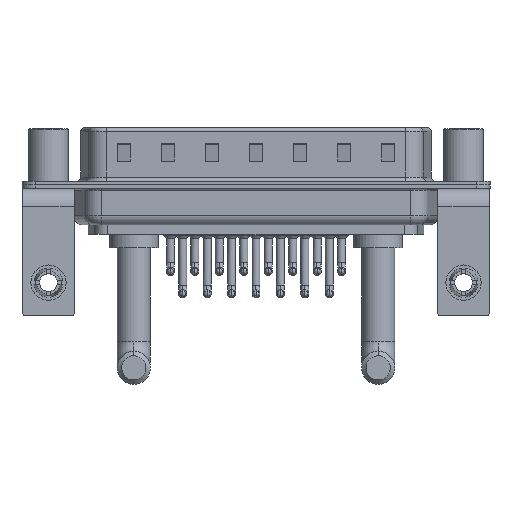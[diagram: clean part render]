
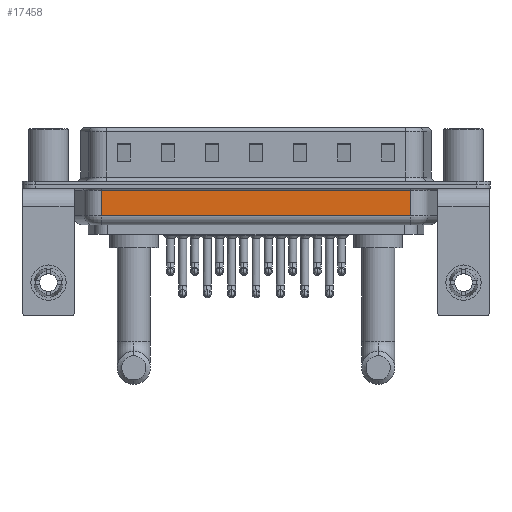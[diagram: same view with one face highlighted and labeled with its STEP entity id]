
A CAD part, front view. The second image highlights one B-rep face of the part: STEP entity #17458.
In plain terms, the highlighted planar face has unit normal (0, -1, 0).
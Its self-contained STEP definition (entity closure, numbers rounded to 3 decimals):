
#133 = LINE ( 'NONE', #23718, #7678 ) ;
#480 = CARTESIAN_POINT ( 'NONE',  ( 6.006, -5.35, -4.5 ) ) ;
#518 = CARTESIAN_POINT ( 'NONE',  ( 41.044, -5.35, -3.5 ) ) ;
#692 = VERTEX_POINT ( 'NONE', #19243 ) ;
#1671 = VECTOR ( 'NONE', #14717, 1000. ) ;
#2708 = VERTEX_POINT ( 'NONE', #16312 ) ;
#3236 = AXIS2_PLACEMENT_3D ( 'NONE', #26106, #8802, #17519 ) ;
#3366 = EDGE_LOOP ( 'NONE', ( #18526, #5207, #11233, #5234 ) ) ;
#4240 = FACE_OUTER_BOUND ( 'NONE', #3366, .T. ) ;
#4291 = DIRECTION ( 'NONE',  ( 1., 0., 0. ) ) ;
#5139 = VERTEX_POINT ( 'NONE', #518 ) ;
#5207 = ORIENTED_EDGE ( 'NONE', *, *, #7796, .T. ) ;
#5234 = ORIENTED_EDGE ( 'NONE', *, *, #7615, .T. ) ;
#6622 = VERTEX_POINT ( 'NONE', #27382 ) ;
#7615 = EDGE_CURVE ( 'NONE', #2708, #692, #10151, .T. ) ;
#7678 = VECTOR ( 'NONE', #4291, 1000. ) ;
#7796 = EDGE_CURVE ( 'NONE', #6622, #5139, #133, .T. ) ;
#7885 = CARTESIAN_POINT ( 'NONE',  ( 41.044, -5.35, -4.5 ) ) ;
#8601 = DIRECTION ( 'NONE',  ( 0., 0., 1. ) ) ;
#8802 = DIRECTION ( 'NONE',  ( 0., 1., 0. ) ) ;
#10151 = LINE ( 'NONE', #21297, #1671 ) ;
#10825 = PLANE ( 'NONE',  #3236 ) ;
#11233 = ORIENTED_EDGE ( 'NONE', *, *, #19568, .T. ) ;
#14048 = LINE ( 'NONE', #480, #23094 ) ;
#14717 = DIRECTION ( 'NONE',  ( -1., 0., 0. ) ) ;
#16312 = CARTESIAN_POINT ( 'NONE',  ( 41.044, -5.35, -0.65 ) ) ;
#17458 = ADVANCED_FACE ( 'NONE', ( #4240 ), #10825, .F. ) ;
#17519 = DIRECTION ( 'NONE',  ( 0., 0., 1. ) ) ;
#18526 = ORIENTED_EDGE ( 'NONE', *, *, #23560, .F. ) ;
#19243 = CARTESIAN_POINT ( 'NONE',  ( 6.006, -5.35, -0.65 ) ) ;
#19258 = VECTOR ( 'NONE', #8601, 1000. ) ;
#19568 = EDGE_CURVE ( 'NONE', #5139, #2708, #23016, .T. ) ;
#21297 = CARTESIAN_POINT ( 'NONE',  ( 6.006, -5.35, -0.65 ) ) ;
#22760 = DIRECTION ( 'NONE',  ( 0., 0., 1. ) ) ;
#23016 = LINE ( 'NONE', #7885, #19258 ) ;
#23094 = VECTOR ( 'NONE', #22760, 1000. ) ;
#23560 = EDGE_CURVE ( 'NONE', #6622, #692, #14048, .T. ) ;
#23718 = CARTESIAN_POINT ( 'NONE',  ( 6.006, -5.35, -3.5 ) ) ;
#26106 = CARTESIAN_POINT ( 'NONE',  ( 6.006, -5.35, -4.5 ) ) ;
#27382 = CARTESIAN_POINT ( 'NONE',  ( 6.006, -5.35, -3.5 ) ) ;
